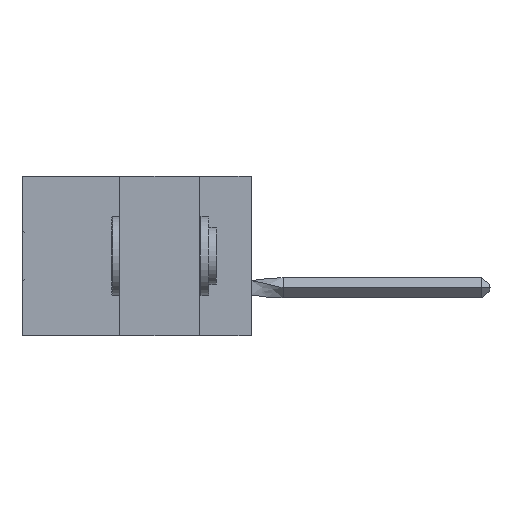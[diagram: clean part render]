
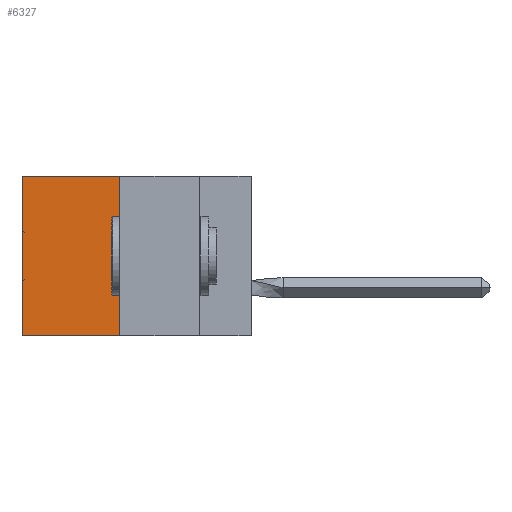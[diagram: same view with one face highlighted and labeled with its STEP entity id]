
A CAD part, left-side view. The second image highlights one B-rep face of the part: STEP entity #6327.
In plain terms, the highlighted planar face has unit normal (-1, 0, 0).
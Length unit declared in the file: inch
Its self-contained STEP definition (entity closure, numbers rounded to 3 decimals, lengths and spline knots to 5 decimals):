
#1547 = EDGE_CURVE ( 'NONE', #3815, #2628, #50454, .T. ) ;
#2628 = VERTEX_POINT ( 'NONE', #48757 ) ;
#3815 = VERTEX_POINT ( 'NONE', #42274 ) ;
#4167 = FACE_OUTER_BOUND ( 'NONE', #38998, .T. ) ;
#5971 = VERTEX_POINT ( 'NONE', #37305 ) ;
#6327 = ADVANCED_FACE ( 'NONE', ( #4167 ), #39910, .F. ) ;
#8683 = DIRECTION ( 'NONE',  ( 0., 0., -1. ) ) ;
#11533 = CARTESIAN_POINT ( 'NONE',  ( 0.305, 0.413, -0.5 ) ) ;
#14368 = ORIENTED_EDGE ( 'NONE', *, *, #37363, .F. ) ;
#15730 = VECTOR ( 'NONE', #35299, 39.37008 ) ;
#18682 = ORIENTED_EDGE ( 'NONE', *, *, #41183, .T. ) ;
#20167 = ORIENTED_EDGE ( 'NONE', *, *, #1547, .T. ) ;
#23968 = LINE ( 'NONE', #31209, #15730 ) ;
#24153 = CARTESIAN_POINT ( 'NONE',  ( 0.305, 0.72, -0.5 ) ) ;
#26747 = VERTEX_POINT ( 'NONE', #42787 ) ;
#30584 = EDGE_CURVE ( 'NONE', #3815, #26747, #23968, .T. ) ;
#31209 = CARTESIAN_POINT ( 'NONE',  ( 0.305, 0.413, -0.5 ) ) ;
#31899 = DIRECTION ( 'NONE',  ( 0., 1., 0. ) ) ;
#32561 = VECTOR ( 'NONE', #40759, 39.37008 ) ;
#32896 = ORIENTED_EDGE ( 'NONE', *, *, #30584, .F. ) ;
#35299 = DIRECTION ( 'NONE',  ( 0., 0., -1. ) ) ;
#35496 = CARTESIAN_POINT ( 'NONE',  ( 0.305, 0.413, 0. ) ) ;
#37010 = DIRECTION ( 'NONE',  ( 1., 0., 0. ) ) ;
#37305 = CARTESIAN_POINT ( 'NONE',  ( 0.305, 0.72, -0.5 ) ) ;
#37363 = EDGE_CURVE ( 'NONE', #26747, #5971, #46316, .T. ) ;
#38998 = EDGE_LOOP ( 'NONE', ( #18682, #14368, #32896, #20167 ) ) ;
#39910 = PLANE ( 'NONE',  #52140 ) ;
#40759 = DIRECTION ( 'NONE',  ( 0., 1., 0. ) ) ;
#40895 = LINE ( 'NONE', #24153, #51087 ) ;
#41183 = EDGE_CURVE ( 'NONE', #2628, #5971, #40895, .T. ) ;
#41233 = VECTOR ( 'NONE', #31899, 39.37008 ) ;
#42274 = CARTESIAN_POINT ( 'NONE',  ( 0.305, 0.413, 0. ) ) ;
#42787 = CARTESIAN_POINT ( 'NONE',  ( 0.305, 0.413, -0.5 ) ) ;
#44148 = CARTESIAN_POINT ( 'NONE',  ( 0.305, 0.413, -0.5 ) ) ;
#46316 = LINE ( 'NONE', #11533, #41233 ) ;
#48757 = CARTESIAN_POINT ( 'NONE',  ( 0.305, 0.72, 0. ) ) ;
#48759 = DIRECTION ( 'NONE',  ( 0., 0., -1. ) ) ;
#50454 = LINE ( 'NONE', #35496, #32561 ) ;
#51087 = VECTOR ( 'NONE', #48759, 39.37008 ) ;
#52140 = AXIS2_PLACEMENT_3D ( 'NONE', #44148, #37010, #8683 ) ;
